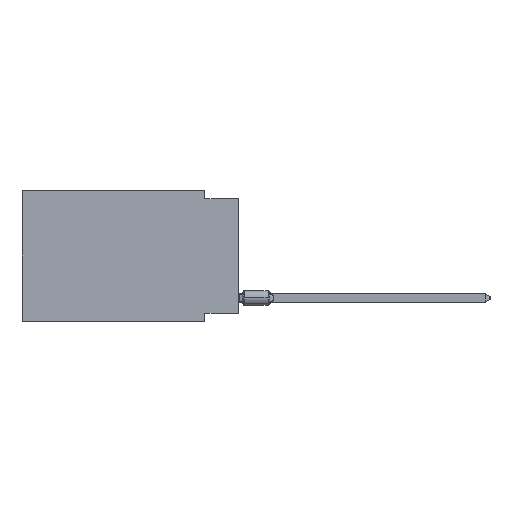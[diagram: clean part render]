
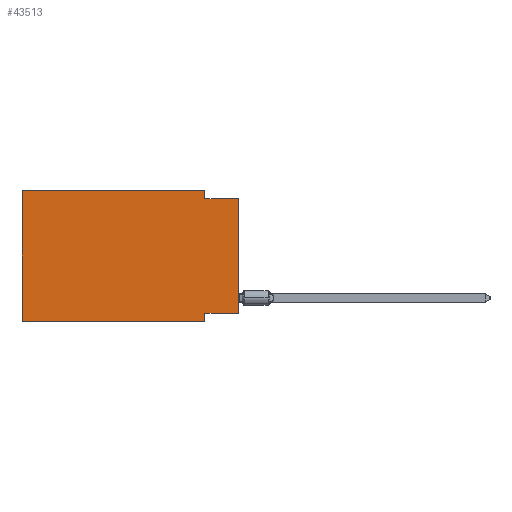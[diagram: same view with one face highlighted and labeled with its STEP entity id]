
A CAD part, left-side view. The second image highlights one B-rep face of the part: STEP entity #43513.
In plain terms, the highlighted planar face has unit normal (-1, 0, 0).
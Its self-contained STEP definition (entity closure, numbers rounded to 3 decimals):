
#2685 = LINE ( 'NONE', #44435, #67367 ) ;
#4374 = VECTOR ( 'NONE', #12590, 1000. ) ;
#5920 = DIRECTION ( 'NONE',  ( 1., 0., 0. ) ) ;
#7856 = VERTEX_POINT ( 'NONE', #22300 ) ;
#10748 = DIRECTION ( 'NONE',  ( 0., 0., -1. ) ) ;
#11222 = DIRECTION ( 'NONE',  ( 0., -1., 0. ) ) ;
#12492 = CARTESIAN_POINT ( 'NONE',  ( 0., 16.383, 0. ) ) ;
#12590 = DIRECTION ( 'NONE',  ( 0., 1., 0. ) ) ;
#13890 = CARTESIAN_POINT ( 'NONE',  ( 0., 2.54, -9.906 ) ) ;
#15915 = ORIENTED_EDGE ( 'NONE', *, *, #66557, .T. ) ;
#16880 = CARTESIAN_POINT ( 'NONE',  ( 0., 16.383, -9.906 ) ) ;
#17804 = DIRECTION ( 'NONE',  ( 0., 0., -1. ) ) ;
#18036 = LINE ( 'NONE', #59017, #4374 ) ;
#18485 = EDGE_CURVE ( 'NONE', #7856, #36006, #57647, .T. ) ;
#19058 = DIRECTION ( 'NONE',  ( 0., -1., 0. ) ) ;
#19383 = VERTEX_POINT ( 'NONE', #53160 ) ;
#19433 = VERTEX_POINT ( 'NONE', #62094 ) ;
#19550 = ORIENTED_EDGE ( 'NONE', *, *, #54815, .T. ) ;
#20932 = EDGE_CURVE ( 'NONE', #63720, #19383, #41392, .T. ) ;
#21755 = CARTESIAN_POINT ( 'NONE',  ( 0., 0., -0.635 ) ) ;
#22300 = CARTESIAN_POINT ( 'NONE',  ( 0., 2.54, -0.635 ) ) ;
#24080 = EDGE_CURVE ( 'NONE', #57309, #53990, #58330, .T. ) ;
#24580 = ORIENTED_EDGE ( 'NONE', *, *, #76009, .F. ) ;
#27899 = CARTESIAN_POINT ( 'NONE',  ( 0., 2.54, -9.906 ) ) ;
#28866 = DIRECTION ( 'NONE',  ( 0., -1., 0. ) ) ;
#29617 = VECTOR ( 'NONE', #36225, 1000. ) ;
#30446 = DIRECTION ( 'NONE',  ( 0., 0., -1. ) ) ;
#31273 = LINE ( 'NONE', #43402, #37869 ) ;
#33749 = VERTEX_POINT ( 'NONE', #16880 ) ;
#35703 = VECTOR ( 'NONE', #17804, 1000. ) ;
#36006 = VERTEX_POINT ( 'NONE', #67401 ) ;
#36225 = DIRECTION ( 'NONE',  ( 0., 0., 1. ) ) ;
#36608 = VECTOR ( 'NONE', #11222, 1000. ) ;
#36957 = EDGE_CURVE ( 'NONE', #33749, #63720, #71728, .T. ) ;
#37869 = VECTOR ( 'NONE', #53935, 1000. ) ;
#38568 = CARTESIAN_POINT ( 'NONE',  ( 0., 16.383, 0. ) ) ;
#41392 = LINE ( 'NONE', #12492, #41779 ) ;
#41779 = VECTOR ( 'NONE', #28866, 1000. ) ;
#42020 = CARTESIAN_POINT ( 'NONE',  ( 0., 2.54, 0. ) ) ;
#42853 = CARTESIAN_POINT ( 'NONE',  ( 0., 16.383, 0. ) ) ;
#43402 = CARTESIAN_POINT ( 'NONE',  ( 0., 0., 0. ) ) ;
#43513 = ADVANCED_FACE ( 'NONE', ( #59323 ), #58950, .F. ) ;
#44435 = CARTESIAN_POINT ( 'NONE',  ( 0., 16.383, -9.906 ) ) ;
#44714 = EDGE_LOOP ( 'NONE', ( #15915, #48568, #51282, #73720, #60071, #19550, #67396, #24580 ) ) ;
#45805 = VECTOR ( 'NONE', #10748, 1000. ) ;
#48568 = ORIENTED_EDGE ( 'NONE', *, *, #18485, .F. ) ;
#48632 = LINE ( 'NONE', #42020, #35703 ) ;
#50129 = CARTESIAN_POINT ( 'NONE',  ( 0., 2.54, -9.271 ) ) ;
#51282 = ORIENTED_EDGE ( 'NONE', *, *, #69674, .F. ) ;
#53160 = CARTESIAN_POINT ( 'NONE',  ( 0., 2.54, 0. ) ) ;
#53935 = DIRECTION ( 'NONE',  ( 0., 0., 1. ) ) ;
#53990 = VERTEX_POINT ( 'NONE', #13890 ) ;
#54815 = EDGE_CURVE ( 'NONE', #33749, #53990, #2685, .T. ) ;
#57309 = VERTEX_POINT ( 'NONE', #50129 ) ;
#57647 = LINE ( 'NONE', #21755, #36608 ) ;
#58330 = LINE ( 'NONE', #27899, #45805 ) ;
#58950 = PLANE ( 'NONE',  #66414 ) ;
#59017 = CARTESIAN_POINT ( 'NONE',  ( 0., 0., -9.271 ) ) ;
#59323 = FACE_OUTER_BOUND ( 'NONE', #44714, .T. ) ;
#60071 = ORIENTED_EDGE ( 'NONE', *, *, #36957, .F. ) ;
#62094 = CARTESIAN_POINT ( 'NONE',  ( 0., 0., -9.271 ) ) ;
#63720 = VERTEX_POINT ( 'NONE', #38568 ) ;
#65983 = CARTESIAN_POINT ( 'NONE',  ( 0., 16.383, 0. ) ) ;
#66414 = AXIS2_PLACEMENT_3D ( 'NONE', #65983, #5920, #30446 ) ;
#66557 = EDGE_CURVE ( 'NONE', #19433, #36006, #31273, .T. ) ;
#67367 = VECTOR ( 'NONE', #19058, 1000. ) ;
#67396 = ORIENTED_EDGE ( 'NONE', *, *, #24080, .F. ) ;
#67401 = CARTESIAN_POINT ( 'NONE',  ( 0., 0., -0.635 ) ) ;
#69674 = EDGE_CURVE ( 'NONE', #19383, #7856, #48632, .T. ) ;
#71728 = LINE ( 'NONE', #42853, #29617 ) ;
#73720 = ORIENTED_EDGE ( 'NONE', *, *, #20932, .F. ) ;
#76009 = EDGE_CURVE ( 'NONE', #19433, #57309, #18036, .T. ) ;
